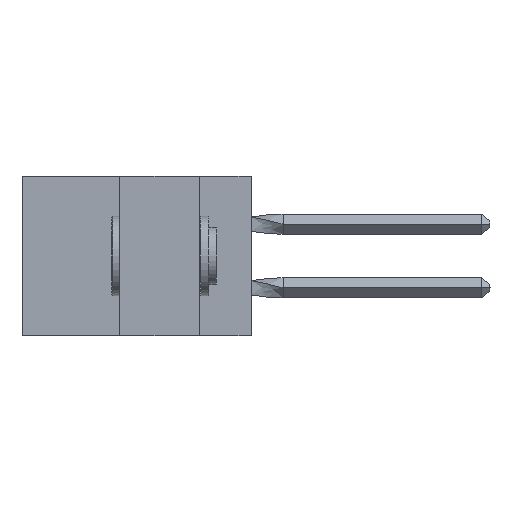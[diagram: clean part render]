
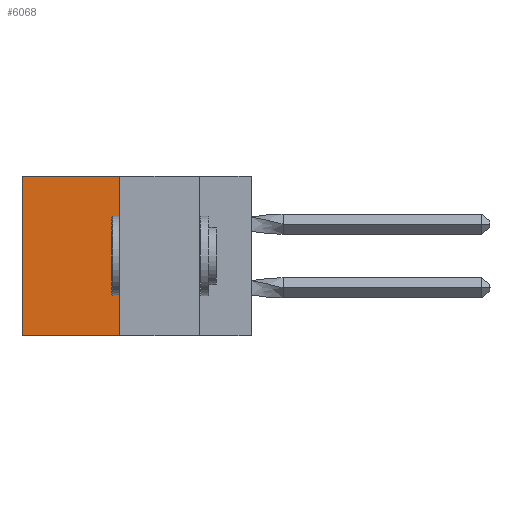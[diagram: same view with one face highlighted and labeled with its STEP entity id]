
A CAD part, left-side view. The second image highlights one B-rep face of the part: STEP entity #6068.
In plain terms, the highlighted planar face has unit normal (-1, 0, 0).
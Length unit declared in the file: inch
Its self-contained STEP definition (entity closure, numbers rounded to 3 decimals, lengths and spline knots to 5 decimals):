
#95 = VERTEX_POINT ( 'NONE', #4668 ) ;
#579 = ORIENTED_EDGE ( 'NONE', *, *, #1275, .F. ) ;
#627 = VERTEX_POINT ( 'NONE', #4396 ) ;
#1143 = ORIENTED_EDGE ( 'NONE', *, *, #8751, .F. ) ;
#1275 = EDGE_CURVE ( 'NONE', #627, #4081, #14972, .T. ) ;
#1289 = DIRECTION ( 'NONE',  ( 0., 1., 0. ) ) ;
#1325 = ORIENTED_EDGE ( 'NONE', *, *, #10014, .T. ) ;
#1432 = DIRECTION ( 'NONE',  ( 1., 0., 0. ) ) ;
#1545 = CARTESIAN_POINT ( 'NONE',  ( 0.305, 0.413, -0.5 ) ) ;
#1901 = LINE ( 'NONE', #4261, #10728 ) ;
#3031 = VERTEX_POINT ( 'NONE', #4793 ) ;
#3340 = EDGE_LOOP ( 'NONE', ( #13491, #1143, #579, #1325 ) ) ;
#3366 = VECTOR ( 'NONE', #9074, 39.37008 ) ;
#4081 = VERTEX_POINT ( 'NONE', #11743 ) ;
#4261 = CARTESIAN_POINT ( 'NONE',  ( 0.305, 0.72, -0.5 ) ) ;
#4323 = LINE ( 'NONE', #15127, #3366 ) ;
#4396 = CARTESIAN_POINT ( 'NONE',  ( 0.305, 0.413, 0. ) ) ;
#4528 = LINE ( 'NONE', #13571, #5869 ) ;
#4668 = CARTESIAN_POINT ( 'NONE',  ( 0.305, 0.72, 0. ) ) ;
#4793 = CARTESIAN_POINT ( 'NONE',  ( 0.305, 0.72, -0.5 ) ) ;
#5869 = VECTOR ( 'NONE', #1289, 39.37008 ) ;
#6068 = ADVANCED_FACE ( 'NONE', ( #8676 ), #13353, .F. ) ;
#6247 = DIRECTION ( 'NONE',  ( 0., 0., -1. ) ) ;
#8676 = FACE_OUTER_BOUND ( 'NONE', #3340, .T. ) ;
#8751 = EDGE_CURVE ( 'NONE', #4081, #3031, #4528, .T. ) ;
#9002 = EDGE_CURVE ( 'NONE', #95, #3031, #1901, .T. ) ;
#9074 = DIRECTION ( 'NONE',  ( 0., 1., 0. ) ) ;
#10014 = EDGE_CURVE ( 'NONE', #627, #95, #4323, .T. ) ;
#10728 = VECTOR ( 'NONE', #15175, 39.37008 ) ;
#11743 = CARTESIAN_POINT ( 'NONE',  ( 0.305, 0.413, -0.5 ) ) ;
#12291 = AXIS2_PLACEMENT_3D ( 'NONE', #1545, #1432, #6247 ) ;
#12756 = DIRECTION ( 'NONE',  ( 0., 0., -1. ) ) ;
#13353 = PLANE ( 'NONE',  #12291 ) ;
#13491 = ORIENTED_EDGE ( 'NONE', *, *, #9002, .T. ) ;
#13571 = CARTESIAN_POINT ( 'NONE',  ( 0.305, 0.413, -0.5 ) ) ;
#13914 = CARTESIAN_POINT ( 'NONE',  ( 0.305, 0.413, -0.5 ) ) ;
#13932 = VECTOR ( 'NONE', #12756, 39.37008 ) ;
#14972 = LINE ( 'NONE', #13914, #13932 ) ;
#15127 = CARTESIAN_POINT ( 'NONE',  ( 0.305, 0.413, 0. ) ) ;
#15175 = DIRECTION ( 'NONE',  ( 0., 0., -1. ) ) ;
